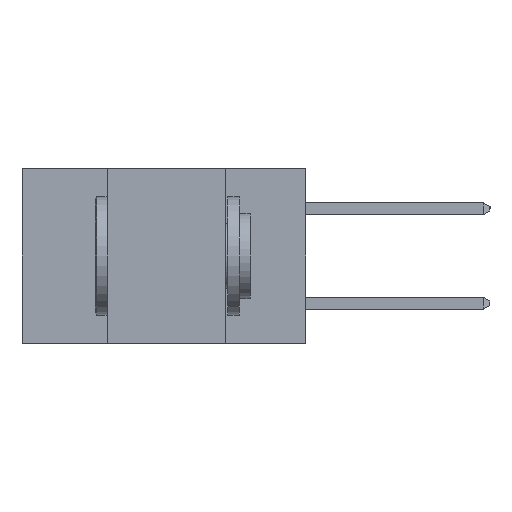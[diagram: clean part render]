
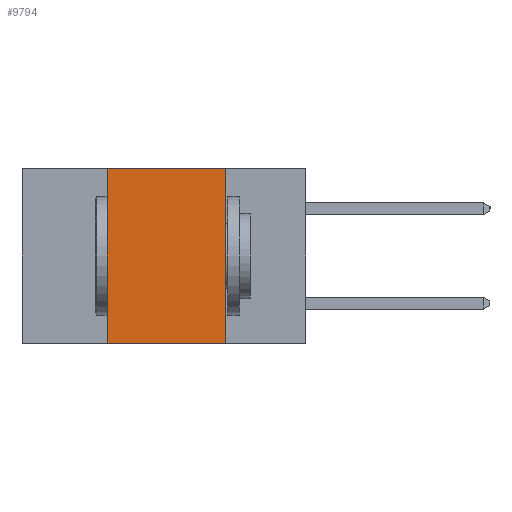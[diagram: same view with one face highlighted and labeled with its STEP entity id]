
A CAD part, left-side view. The second image highlights one B-rep face of the part: STEP entity #9794.
In plain terms, the highlighted planar face has unit normal (-1, 0, 0).
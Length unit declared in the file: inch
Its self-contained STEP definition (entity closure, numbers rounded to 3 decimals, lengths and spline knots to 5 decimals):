
#264 = LINE ( 'NONE', #897, #437 ) ;
#397 = VECTOR ( 'NONE', #2271, 39.37008 ) ;
#437 = VECTOR ( 'NONE', #1066, 39.37008 ) ;
#897 = CARTESIAN_POINT ( 'NONE',  ( 0., 0.17, -0.37 ) ) ;
#1066 = DIRECTION ( 'NONE',  ( 0., 0., -1. ) ) ;
#1179 = EDGE_CURVE ( 'NONE', #7113, #5399, #10339, .T. ) ;
#1199 = CARTESIAN_POINT ( 'NONE',  ( 0., 0.17, -0.37 ) ) ;
#1624 = FACE_OUTER_BOUND ( 'NONE', #8710, .T. ) ;
#1974 = AXIS2_PLACEMENT_3D ( 'NONE', #3311, #6938, #3476 ) ;
#2256 = EDGE_CURVE ( 'NONE', #4981, #6224, #264, .T. ) ;
#2271 = DIRECTION ( 'NONE',  ( 0., 0., 1. ) ) ;
#2630 = LINE ( 'NONE', #9617, #4280 ) ;
#3252 = PLANE ( 'NONE',  #1974 ) ;
#3311 = CARTESIAN_POINT ( 'NONE',  ( 0., 0.6, 0. ) ) ;
#3476 = DIRECTION ( 'NONE',  ( 0., 0., -1. ) ) ;
#4280 = VECTOR ( 'NONE', #10590, 39.37008 ) ;
#4938 = VECTOR ( 'NONE', #7810, 39.37008 ) ;
#4978 = CARTESIAN_POINT ( 'NONE',  ( 0., 0.42, -0.37 ) ) ;
#4981 = VERTEX_POINT ( 'NONE', #9208 ) ;
#5046 = CARTESIAN_POINT ( 'NONE',  ( 0., 0.6, -0.37 ) ) ;
#5399 = VERTEX_POINT ( 'NONE', #6368 ) ;
#6224 = VERTEX_POINT ( 'NONE', #1199 ) ;
#6368 = CARTESIAN_POINT ( 'NONE',  ( 0., 0.42, 0. ) ) ;
#6938 = DIRECTION ( 'NONE',  ( 1., 0., 0. ) ) ;
#7113 = VERTEX_POINT ( 'NONE', #10100 ) ;
#7501 = ORIENTED_EDGE ( 'NONE', *, *, #7895, .F. ) ;
#7810 = DIRECTION ( 'NONE',  ( 0., -1., 0. ) ) ;
#7895 = EDGE_CURVE ( 'NONE', #5399, #4981, #2630, .T. ) ;
#8441 = ORIENTED_EDGE ( 'NONE', *, *, #9705, .T. ) ;
#8710 = EDGE_LOOP ( 'NONE', ( #8810, #7501, #10469, #8441 ) ) ;
#8810 = ORIENTED_EDGE ( 'NONE', *, *, #2256, .F. ) ;
#9208 = CARTESIAN_POINT ( 'NONE',  ( 0., 0.17, 0. ) ) ;
#9617 = CARTESIAN_POINT ( 'NONE',  ( 0., 0.6, 0. ) ) ;
#9705 = EDGE_CURVE ( 'NONE', #7113, #6224, #10512, .T. ) ;
#9794 = ADVANCED_FACE ( 'NONE', ( #1624 ), #3252, .F. ) ;
#10100 = CARTESIAN_POINT ( 'NONE',  ( 0., 0.42, -0.37 ) ) ;
#10339 = LINE ( 'NONE', #4978, #397 ) ;
#10469 = ORIENTED_EDGE ( 'NONE', *, *, #1179, .F. ) ;
#10512 = LINE ( 'NONE', #5046, #4938 ) ;
#10590 = DIRECTION ( 'NONE',  ( 0., -1., 0. ) ) ;
